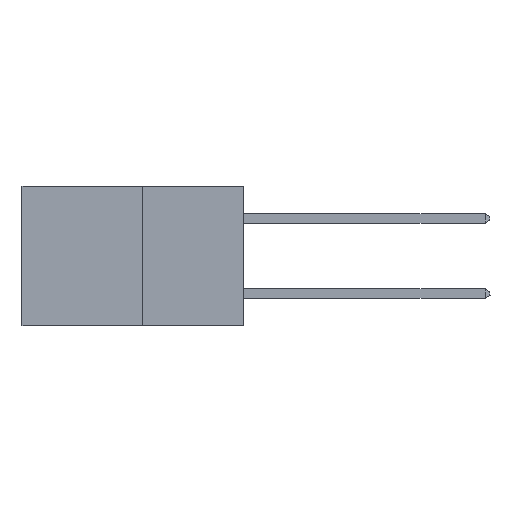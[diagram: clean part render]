
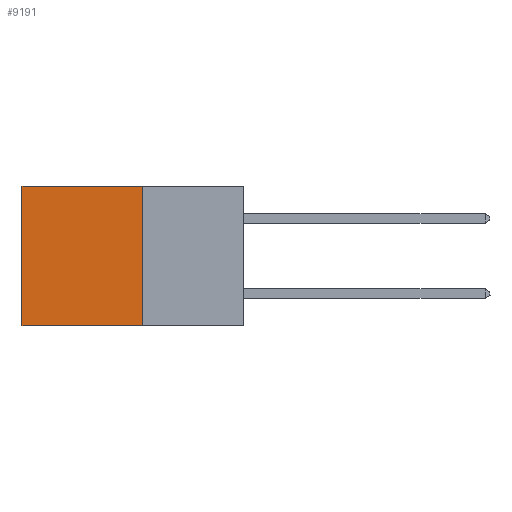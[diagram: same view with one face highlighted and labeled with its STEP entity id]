
A CAD part, left-side view. The second image highlights one B-rep face of the part: STEP entity #9191.
In plain terms, the highlighted planar face has unit normal (-1, 0, 0).
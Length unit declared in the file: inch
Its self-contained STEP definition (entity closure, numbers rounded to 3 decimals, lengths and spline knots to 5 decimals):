
#541 = LINE ( 'NONE', #1603, #10623 ) ;
#1096 = AXIS2_PLACEMENT_3D ( 'NONE', #5883, #9842, #3962 ) ;
#1466 = CARTESIAN_POINT ( 'NONE',  ( 0.277, 0.59, -0.37 ) ) ;
#1603 = CARTESIAN_POINT ( 'NONE',  ( 0.277, 0.27, -0.37 ) ) ;
#1933 = EDGE_CURVE ( 'NONE', #11326, #6895, #10702, .T. ) ;
#2965 = EDGE_CURVE ( 'NONE', #10465, #6895, #9493, .T. ) ;
#3204 = ORIENTED_EDGE ( 'NONE', *, *, #1933, .T. ) ;
#3962 = DIRECTION ( 'NONE',  ( 0., 0., -1. ) ) ;
#4159 = CARTESIAN_POINT ( 'NONE',  ( 0.277, 0.27, -0.37 ) ) ;
#4473 = FACE_OUTER_BOUND ( 'NONE', #6416, .T. ) ;
#4554 = CARTESIAN_POINT ( 'NONE',  ( 0.277, 0.27, 0. ) ) ;
#5017 = DIRECTION ( 'NONE',  ( 0., 1., 0. ) ) ;
#5034 = EDGE_CURVE ( 'NONE', #9756, #10465, #541, .T. ) ;
#5200 = VECTOR ( 'NONE', #9279, 39.37008 ) ;
#5452 = DIRECTION ( 'NONE',  ( 0., 1., 0. ) ) ;
#5676 = LINE ( 'NONE', #4554, #7412 ) ;
#5685 = CARTESIAN_POINT ( 'NONE',  ( 0.277, 0.27, 0. ) ) ;
#5883 = CARTESIAN_POINT ( 'NONE',  ( 0.277, 0.27, -0.37 ) ) ;
#6416 = EDGE_LOOP ( 'NONE', ( #3204, #10523, #9927, #11670 ) ) ;
#6512 = EDGE_CURVE ( 'NONE', #9756, #11326, #5676, .T. ) ;
#6548 = VECTOR ( 'NONE', #5017, 39.37008 ) ;
#6704 = CARTESIAN_POINT ( 'NONE',  ( 0.277, 0.27, -0.37 ) ) ;
#6895 = VERTEX_POINT ( 'NONE', #1466 ) ;
#7412 = VECTOR ( 'NONE', #5452, 39.37008 ) ;
#8846 = PLANE ( 'NONE',  #1096 ) ;
#9191 = ADVANCED_FACE ( 'NONE', ( #4473 ), #8846, .F. ) ;
#9279 = DIRECTION ( 'NONE',  ( 0., 0., -1. ) ) ;
#9342 = DIRECTION ( 'NONE',  ( 0., 0., -1. ) ) ;
#9364 = CARTESIAN_POINT ( 'NONE',  ( 0.277, 0.59, -0.37 ) ) ;
#9493 = LINE ( 'NONE', #4159, #6548 ) ;
#9756 = VERTEX_POINT ( 'NONE', #5685 ) ;
#9842 = DIRECTION ( 'NONE',  ( 1., 0., 0. ) ) ;
#9927 = ORIENTED_EDGE ( 'NONE', *, *, #5034, .F. ) ;
#10465 = VERTEX_POINT ( 'NONE', #6704 ) ;
#10523 = ORIENTED_EDGE ( 'NONE', *, *, #2965, .F. ) ;
#10623 = VECTOR ( 'NONE', #9342, 39.37008 ) ;
#10702 = LINE ( 'NONE', #9364, #5200 ) ;
#10940 = CARTESIAN_POINT ( 'NONE',  ( 0.277, 0.59, 0. ) ) ;
#11326 = VERTEX_POINT ( 'NONE', #10940 ) ;
#11670 = ORIENTED_EDGE ( 'NONE', *, *, #6512, .T. ) ;
